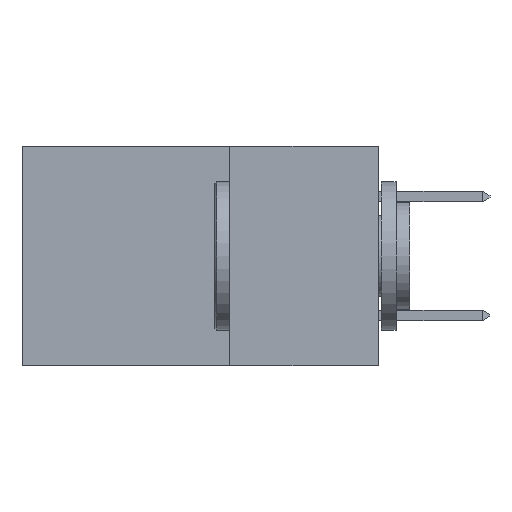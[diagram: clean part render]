
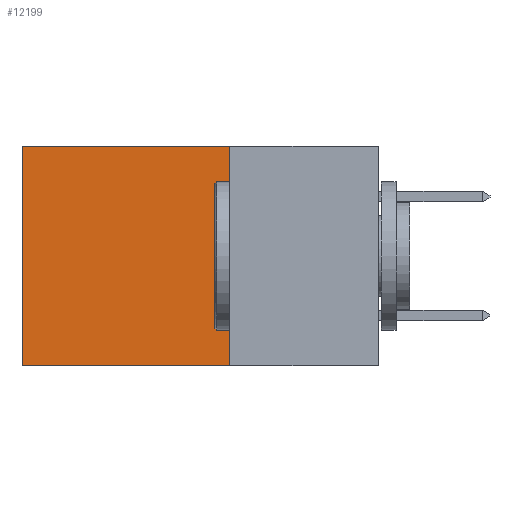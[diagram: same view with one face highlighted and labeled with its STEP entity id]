
A CAD part, left-side view. The second image highlights one B-rep face of the part: STEP entity #12199.
In plain terms, the highlighted planar face has unit normal (-1, 0, 0).
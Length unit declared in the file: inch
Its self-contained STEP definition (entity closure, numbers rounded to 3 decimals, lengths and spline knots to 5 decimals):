
#498 = VECTOR ( 'NONE', #7430, 39.37008 ) ;
#645 = ORIENTED_EDGE ( 'NONE', *, *, #4625, .F. ) ;
#1686 = VECTOR ( 'NONE', #13532, 39.37008 ) ;
#1768 = EDGE_CURVE ( 'NONE', #2583, #8658, #7314, .T. ) ;
#2285 = CARTESIAN_POINT ( 'NONE',  ( 0.298, 0.25, 0. ) ) ;
#2583 = VERTEX_POINT ( 'NONE', #11501 ) ;
#2624 = CARTESIAN_POINT ( 'NONE',  ( 0.298, 0.6, 0. ) ) ;
#3479 = DIRECTION ( 'NONE',  ( 0., 0., -1. ) ) ;
#3591 = VERTEX_POINT ( 'NONE', #2624 ) ;
#3856 = ORIENTED_EDGE ( 'NONE', *, *, #1768, .F. ) ;
#4070 = LINE ( 'NONE', #11793, #498 ) ;
#4625 = EDGE_CURVE ( 'NONE', #8658, #8552, #12286, .T. ) ;
#5805 = CARTESIAN_POINT ( 'NONE',  ( 0.298, 0.25, -0.37 ) ) ;
#6537 = ORIENTED_EDGE ( 'NONE', *, *, #9925, .T. ) ;
#7314 = LINE ( 'NONE', #9954, #12784 ) ;
#7430 = DIRECTION ( 'NONE',  ( 0., 1., 0. ) ) ;
#7818 = LINE ( 'NONE', #10283, #1686 ) ;
#7951 = FACE_OUTER_BOUND ( 'NONE', #9931, .T. ) ;
#8552 = VERTEX_POINT ( 'NONE', #11138 ) ;
#8554 = DIRECTION ( 'NONE',  ( 0., 1., 0. ) ) ;
#8623 = DIRECTION ( 'NONE',  ( 0., 0., -1. ) ) ;
#8658 = VERTEX_POINT ( 'NONE', #5805 ) ;
#9068 = PLANE ( 'NONE',  #9395 ) ;
#9395 = AXIS2_PLACEMENT_3D ( 'NONE', #2285, #10172, #3479 ) ;
#9925 = EDGE_CURVE ( 'NONE', #3591, #8552, #7818, .T. ) ;
#9931 = EDGE_LOOP ( 'NONE', ( #6537, #645, #3856, #12711 ) ) ;
#9954 = CARTESIAN_POINT ( 'NONE',  ( 0.298, 0.25, 0. ) ) ;
#10172 = DIRECTION ( 'NONE',  ( 1., 0., 0. ) ) ;
#10283 = CARTESIAN_POINT ( 'NONE',  ( 0.298, 0.6, 0. ) ) ;
#11138 = CARTESIAN_POINT ( 'NONE',  ( 0.298, 0.6, -0.37 ) ) ;
#11157 = EDGE_CURVE ( 'NONE', #2583, #3591, #4070, .T. ) ;
#11501 = CARTESIAN_POINT ( 'NONE',  ( 0.298, 0.25, 0. ) ) ;
#11793 = CARTESIAN_POINT ( 'NONE',  ( 0.298, 0.25, 0. ) ) ;
#12199 = ADVANCED_FACE ( 'NONE', ( #7951 ), #9068, .F. ) ;
#12286 = LINE ( 'NONE', #13224, #14413 ) ;
#12711 = ORIENTED_EDGE ( 'NONE', *, *, #11157, .T. ) ;
#12784 = VECTOR ( 'NONE', #8623, 39.37008 ) ;
#13224 = CARTESIAN_POINT ( 'NONE',  ( 0.298, 0.25, -0.37 ) ) ;
#13532 = DIRECTION ( 'NONE',  ( 0., 0., -1. ) ) ;
#14413 = VECTOR ( 'NONE', #8554, 39.37008 ) ;
